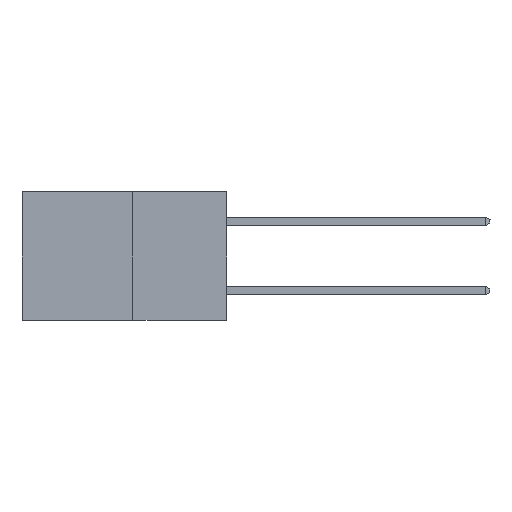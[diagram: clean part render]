
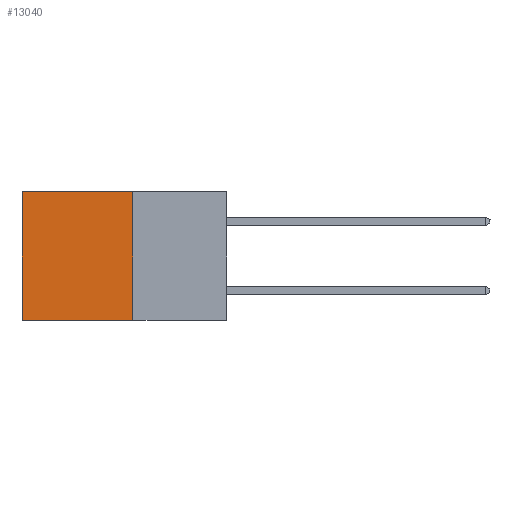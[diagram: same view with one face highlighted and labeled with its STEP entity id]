
A CAD part, left-side view. The second image highlights one B-rep face of the part: STEP entity #13040.
In plain terms, the highlighted planar face has unit normal (-1, 0, 0).
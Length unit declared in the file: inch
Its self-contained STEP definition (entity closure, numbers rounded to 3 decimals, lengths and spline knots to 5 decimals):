
#395 = DIRECTION ( 'NONE',  ( 1., 0., 0. ) ) ;
#1900 = EDGE_CURVE ( 'NONE', #24541, #7599, #20195, .T. ) ;
#2916 = CARTESIAN_POINT ( 'NONE',  ( 0.277, 0.59, -0.37 ) ) ;
#4570 = LINE ( 'NONE', #15717, #20962 ) ;
#6890 = ORIENTED_EDGE ( 'NONE', *, *, #11338, .T. ) ;
#7235 = AXIS2_PLACEMENT_3D ( 'NONE', #8979, #395, #15473 ) ;
#7599 = VERTEX_POINT ( 'NONE', #8792 ) ;
#7624 = CARTESIAN_POINT ( 'NONE',  ( 0.277, 0.27, -0.37 ) ) ;
#8792 = CARTESIAN_POINT ( 'NONE',  ( 0.277, 0.27, -0.37 ) ) ;
#8979 = CARTESIAN_POINT ( 'NONE',  ( 0.277, 0.27, -0.37 ) ) ;
#9081 = VECTOR ( 'NONE', #24847, 39.37008 ) ;
#10112 = DIRECTION ( 'NONE',  ( 0., 0., -1. ) ) ;
#11338 = EDGE_CURVE ( 'NONE', #24541, #12652, #4570, .T. ) ;
#11357 = VERTEX_POINT ( 'NONE', #2916 ) ;
#11482 = CARTESIAN_POINT ( 'NONE',  ( 0.277, 0.27, -0.37 ) ) ;
#12652 = VERTEX_POINT ( 'NONE', #25942 ) ;
#13040 = ADVANCED_FACE ( 'NONE', ( #23477 ), #25949, .F. ) ;
#14807 = LINE ( 'NONE', #16432, #9081 ) ;
#15473 = DIRECTION ( 'NONE',  ( 0., 0., -1. ) ) ;
#15717 = CARTESIAN_POINT ( 'NONE',  ( 0.277, 0.27, 0. ) ) ;
#16111 = VECTOR ( 'NONE', #24625, 39.37008 ) ;
#16295 = ORIENTED_EDGE ( 'NONE', *, *, #1900, .F. ) ;
#16432 = CARTESIAN_POINT ( 'NONE',  ( 0.277, 0.59, -0.37 ) ) ;
#16556 = ORIENTED_EDGE ( 'NONE', *, *, #22941, .F. ) ;
#17511 = ORIENTED_EDGE ( 'NONE', *, *, #26930, .T. ) ;
#17973 = EDGE_LOOP ( 'NONE', ( #17511, #16556, #16295, #6890 ) ) ;
#19903 = DIRECTION ( 'NONE',  ( 0., 1., 0. ) ) ;
#20195 = LINE ( 'NONE', #11482, #25735 ) ;
#20962 = VECTOR ( 'NONE', #19903, 39.37008 ) ;
#21705 = LINE ( 'NONE', #7624, #16111 ) ;
#22941 = EDGE_CURVE ( 'NONE', #7599, #11357, #21705, .T. ) ;
#23477 = FACE_OUTER_BOUND ( 'NONE', #17973, .T. ) ;
#24541 = VERTEX_POINT ( 'NONE', #25782 ) ;
#24625 = DIRECTION ( 'NONE',  ( 0., 1., 0. ) ) ;
#24847 = DIRECTION ( 'NONE',  ( 0., 0., -1. ) ) ;
#25735 = VECTOR ( 'NONE', #10112, 39.37008 ) ;
#25782 = CARTESIAN_POINT ( 'NONE',  ( 0.277, 0.27, 0. ) ) ;
#25942 = CARTESIAN_POINT ( 'NONE',  ( 0.277, 0.59, 0. ) ) ;
#25949 = PLANE ( 'NONE',  #7235 ) ;
#26930 = EDGE_CURVE ( 'NONE', #12652, #11357, #14807, .T. ) ;
